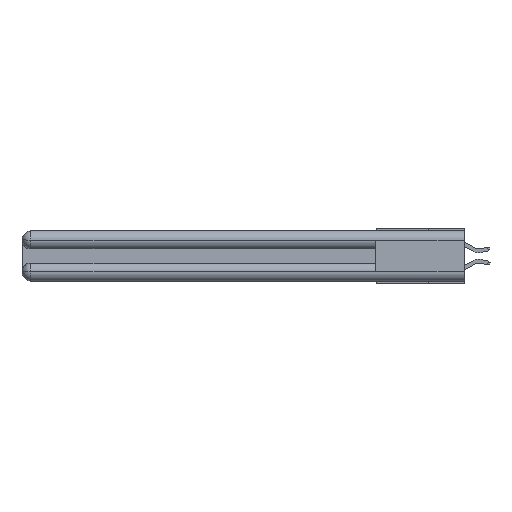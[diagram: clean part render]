
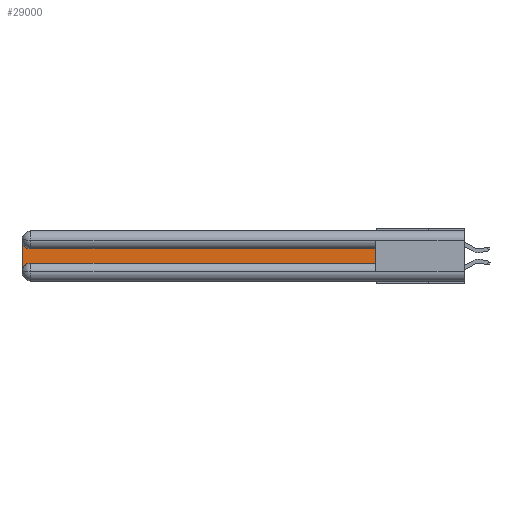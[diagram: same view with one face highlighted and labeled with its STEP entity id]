
A CAD part, left-side view. The second image highlights one B-rep face of the part: STEP entity #29000.
In plain terms, the highlighted planar face has unit normal (-1, 0, 0).
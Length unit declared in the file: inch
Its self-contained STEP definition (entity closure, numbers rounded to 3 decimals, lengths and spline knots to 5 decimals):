
#1572 = CARTESIAN_POINT ( 'NONE',  ( 0.075, 2.94, -0.1225 ) ) ;
#3166 = DIRECTION ( 'NONE',  ( 0., 0., 1. ) ) ;
#4309 = CARTESIAN_POINT ( 'NONE',  ( 0.075, 0.6, -0.2175 ) ) ;
#4361 = DIRECTION ( 'NONE',  ( 1., 0., 0. ) ) ;
#4762 = LINE ( 'NONE', #6198, #16973 ) ;
#4969 = CARTESIAN_POINT ( 'NONE',  ( 0.075, 0.6, -0.1225 ) ) ;
#5328 = CARTESIAN_POINT ( 'NONE',  ( 0.075, 0.6, -0.2175 ) ) ;
#5661 = AXIS2_PLACEMENT_3D ( 'NONE', #24281, #16766, #17582 ) ;
#6028 = CARTESIAN_POINT ( 'NONE',  ( 0.075, 2.94, -0.2175 ) ) ;
#6198 = CARTESIAN_POINT ( 'NONE',  ( 0.075, 0.6, -0.1225 ) ) ;
#6309 = CIRCLE ( 'NONE', #20728, 0.06 ) ;
#6397 = DIRECTION ( 'NONE',  ( 0., 1., 0. ) ) ;
#6421 = DIRECTION ( 'NONE',  ( 0., -1., 0. ) ) ;
#6796 = ORIENTED_EDGE ( 'NONE', *, *, #20523, .T. ) ;
#6935 = CARTESIAN_POINT ( 'NONE',  ( 0.075, 2.94, -0.0625 ) ) ;
#7295 = EDGE_CURVE ( 'NONE', #16494, #27271, #4762, .T. ) ;
#7711 = VECTOR ( 'NONE', #16326, 39.37008 ) ;
#8041 = VERTEX_POINT ( 'NONE', #20275 ) ;
#8749 = VERTEX_POINT ( 'NONE', #23373 ) ;
#9115 = ORIENTED_EDGE ( 'NONE', *, *, #14062, .T. ) ;
#9146 = LINE ( 'NONE', #18773, #7711 ) ;
#11434 = DIRECTION ( 'NONE',  ( 0., 0., -1. ) ) ;
#12872 = EDGE_LOOP ( 'NONE', ( #25485, #9115, #6796, #19030, #25100, #25854 ) ) ;
#13251 = LINE ( 'NONE', #25800, #21531 ) ;
#14062 = EDGE_CURVE ( 'NONE', #27271, #8041, #6309, .T. ) ;
#16326 = DIRECTION ( 'NONE',  ( 0., 0., -1. ) ) ;
#16494 = VERTEX_POINT ( 'NONE', #4969 ) ;
#16766 = DIRECTION ( 'NONE',  ( 1., 0., 0. ) ) ;
#16810 = LINE ( 'NONE', #4309, #20428 ) ;
#16973 = VECTOR ( 'NONE', #6397, 39.37008 ) ;
#17582 = DIRECTION ( 'NONE',  ( 0., 0., -1. ) ) ;
#18037 = PLANE ( 'NONE',  #25710 ) ;
#18133 = CARTESIAN_POINT ( 'NONE',  ( 0.075, 3., -0.1225 ) ) ;
#18234 = DIRECTION ( 'NONE',  ( 0., 0., -1. ) ) ;
#18773 = CARTESIAN_POINT ( 'NONE',  ( 0.075, 3., -0.2175 ) ) ;
#19030 = ORIENTED_EDGE ( 'NONE', *, *, #23936, .T. ) ;
#20275 = CARTESIAN_POINT ( 'NONE',  ( 0.075, 3., -0.0625 ) ) ;
#20333 = FACE_OUTER_BOUND ( 'NONE', #12872, .T. ) ;
#20428 = VECTOR ( 'NONE', #6421, 39.37008 ) ;
#20518 = VERTEX_POINT ( 'NONE', #5328 ) ;
#20523 = EDGE_CURVE ( 'NONE', #8041, #8749, #9146, .T. ) ;
#20728 = AXIS2_PLACEMENT_3D ( 'NONE', #6935, #27269, #11434 ) ;
#20749 = VERTEX_POINT ( 'NONE', #6028 ) ;
#21531 = VECTOR ( 'NONE', #3166, 39.37008 ) ;
#21551 = CIRCLE ( 'NONE', #5661, 0.06 ) ;
#23373 = CARTESIAN_POINT ( 'NONE',  ( 0.075, 3., -0.2775 ) ) ;
#23936 = EDGE_CURVE ( 'NONE', #8749, #20749, #21551, .T. ) ;
#24281 = CARTESIAN_POINT ( 'NONE',  ( 0.075, 2.94, -0.2775 ) ) ;
#24731 = EDGE_CURVE ( 'NONE', #20518, #16494, #13251, .T. ) ;
#25100 = ORIENTED_EDGE ( 'NONE', *, *, #27456, .T. ) ;
#25485 = ORIENTED_EDGE ( 'NONE', *, *, #7295, .T. ) ;
#25710 = AXIS2_PLACEMENT_3D ( 'NONE', #18133, #4361, #18234 ) ;
#25800 = CARTESIAN_POINT ( 'NONE',  ( 0.075, 0.6, -0.2175 ) ) ;
#25854 = ORIENTED_EDGE ( 'NONE', *, *, #24731, .T. ) ;
#27269 = DIRECTION ( 'NONE',  ( 1., 0., 0. ) ) ;
#27271 = VERTEX_POINT ( 'NONE', #1572 ) ;
#27456 = EDGE_CURVE ( 'NONE', #20749, #20518, #16810, .T. ) ;
#29000 = ADVANCED_FACE ( 'NONE', ( #20333 ), #18037, .F. ) ;
